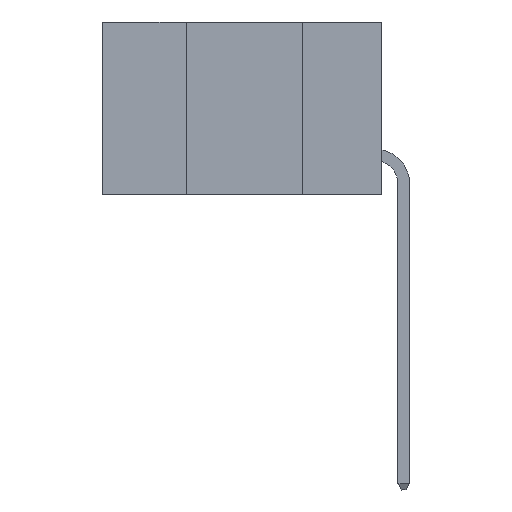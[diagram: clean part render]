
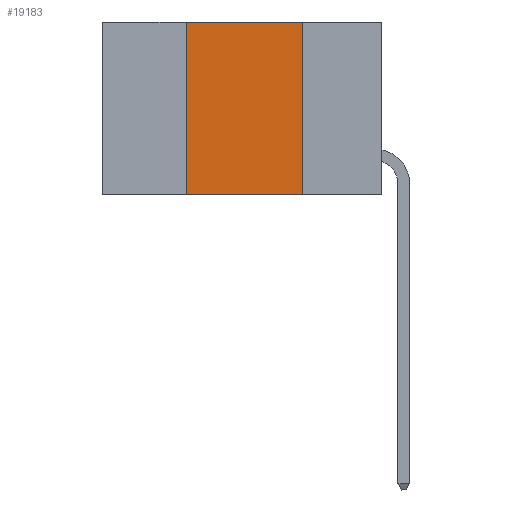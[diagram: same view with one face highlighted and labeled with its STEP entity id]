
A CAD part, left-side view. The second image highlights one B-rep face of the part: STEP entity #19183.
In plain terms, the highlighted planar face has unit normal (-1, 0, 0).
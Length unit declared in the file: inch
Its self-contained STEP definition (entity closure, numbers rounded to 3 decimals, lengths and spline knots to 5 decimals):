
#48 = CARTESIAN_POINT ( 'NONE',  ( 0., 0.42, -0.37 ) ) ;
#500 = ORIENTED_EDGE ( 'NONE', *, *, #4301, .F. ) ;
#1137 = ORIENTED_EDGE ( 'NONE', *, *, #19340, .T. ) ;
#1152 = LINE ( 'NONE', #32264, #31496 ) ;
#3125 = EDGE_LOOP ( 'NONE', ( #26064, #35784, #500, #1137 ) ) ;
#3173 = VECTOR ( 'NONE', #35758, 39.37008 ) ;
#4103 = LINE ( 'NONE', #21189, #3173 ) ;
#4147 = CARTESIAN_POINT ( 'NONE',  ( 0., 0.6, -0.37 ) ) ;
#4301 = EDGE_CURVE ( 'NONE', #4851, #37930, #4103, .T. ) ;
#4851 = VERTEX_POINT ( 'NONE', #48 ) ;
#5014 = LINE ( 'NONE', #4147, #20660 ) ;
#6352 = CARTESIAN_POINT ( 'NONE',  ( 0., 0.6, 0. ) ) ;
#7195 = EDGE_CURVE ( 'NONE', #37930, #28357, #1152, .T. ) ;
#9315 = DIRECTION ( 'NONE',  ( 1., 0., 0. ) ) ;
#9371 = VERTEX_POINT ( 'NONE', #29442 ) ;
#10987 = LINE ( 'NONE', #13961, #31663 ) ;
#13961 = CARTESIAN_POINT ( 'NONE',  ( 0., 0.17, 0. ) ) ;
#18375 = FACE_OUTER_BOUND ( 'NONE', #3125, .T. ) ;
#19183 = ADVANCED_FACE ( 'NONE', ( #18375 ), #23919, .F. ) ;
#19340 = EDGE_CURVE ( 'NONE', #4851, #9371, #5014, .T. ) ;
#20660 = VECTOR ( 'NONE', #21744, 39.37008 ) ;
#21179 = CARTESIAN_POINT ( 'NONE',  ( 0., 0.17, 0. ) ) ;
#21189 = CARTESIAN_POINT ( 'NONE',  ( 0., 0.42, 0. ) ) ;
#21744 = DIRECTION ( 'NONE',  ( 0., -1., 0. ) ) ;
#21761 = AXIS2_PLACEMENT_3D ( 'NONE', #6352, #9315, #29815 ) ;
#23919 = PLANE ( 'NONE',  #21761 ) ;
#26064 = ORIENTED_EDGE ( 'NONE', *, *, #31920, .F. ) ;
#28357 = VERTEX_POINT ( 'NONE', #21179 ) ;
#29442 = CARTESIAN_POINT ( 'NONE',  ( 0., 0.17, -0.37 ) ) ;
#29815 = DIRECTION ( 'NONE',  ( 0., 0., -1. ) ) ;
#31496 = VECTOR ( 'NONE', #35158, 39.37008 ) ;
#31534 = DIRECTION ( 'NONE',  ( 0., 0., -1. ) ) ;
#31663 = VECTOR ( 'NONE', #31534, 39.37008 ) ;
#31920 = EDGE_CURVE ( 'NONE', #28357, #9371, #10987, .T. ) ;
#32264 = CARTESIAN_POINT ( 'NONE',  ( 0., 0.6, 0. ) ) ;
#32952 = CARTESIAN_POINT ( 'NONE',  ( 0., 0.42, 0. ) ) ;
#35158 = DIRECTION ( 'NONE',  ( 0., -1., 0. ) ) ;
#35758 = DIRECTION ( 'NONE',  ( 0., 0., 1. ) ) ;
#35784 = ORIENTED_EDGE ( 'NONE', *, *, #7195, .F. ) ;
#37930 = VERTEX_POINT ( 'NONE', #32952 ) ;
